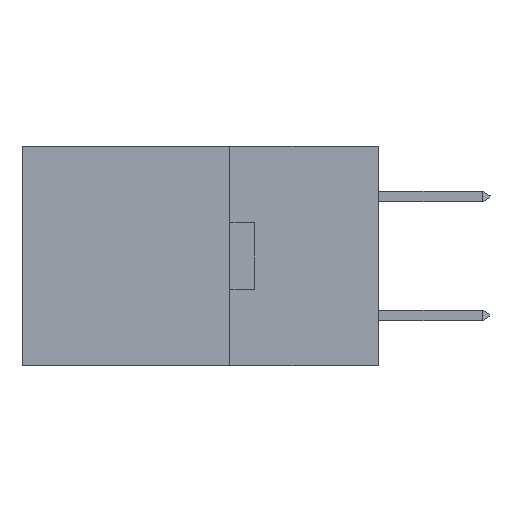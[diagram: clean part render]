
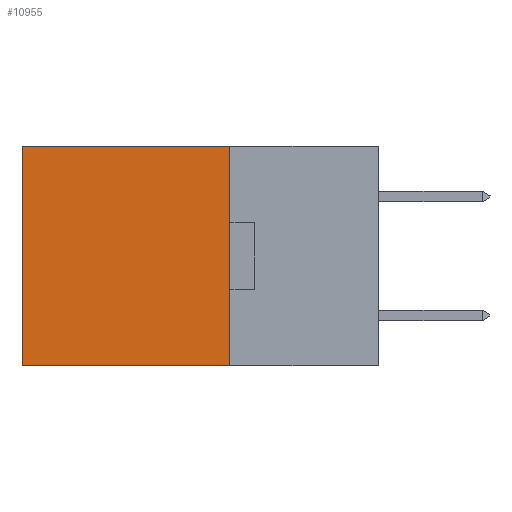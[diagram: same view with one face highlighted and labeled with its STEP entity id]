
A CAD part, left-side view. The second image highlights one B-rep face of the part: STEP entity #10955.
In plain terms, the highlighted planar face has unit normal (-1, 0, 0).
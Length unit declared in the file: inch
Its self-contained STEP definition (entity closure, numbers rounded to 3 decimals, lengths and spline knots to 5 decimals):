
#260 = CARTESIAN_POINT ( 'NONE',  ( 0.2615, 0.6, -0.37 ) ) ;
#2380 = DIRECTION ( 'NONE',  ( 0., 0., -1. ) ) ;
#3137 = CARTESIAN_POINT ( 'NONE',  ( 0.2615, 0.25, -0.37 ) ) ;
#4260 = VECTOR ( 'NONE', #11902, 39.37008 ) ;
#5632 = EDGE_CURVE ( 'NONE', #25134, #18917, #22553, .T. ) ;
#5729 = VECTOR ( 'NONE', #23859, 39.37008 ) ;
#6984 = FACE_OUTER_BOUND ( 'NONE', #23196, .T. ) ;
#8907 = DIRECTION ( 'NONE',  ( 0., 0., -1. ) ) ;
#9344 = ORIENTED_EDGE ( 'NONE', *, *, #13619, .T. ) ;
#9920 = CARTESIAN_POINT ( 'NONE',  ( 0.2615, 0.25, -0.37 ) ) ;
#9975 = ORIENTED_EDGE ( 'NONE', *, *, #25076, .F. ) ;
#10955 = ADVANCED_FACE ( 'NONE', ( #6984 ), #11305, .F. ) ;
#11305 = PLANE ( 'NONE',  #12010 ) ;
#11430 = ORIENTED_EDGE ( 'NONE', *, *, #5632, .T. ) ;
#11448 = CARTESIAN_POINT ( 'NONE',  ( 0.2615, 0.25, -0.37 ) ) ;
#11644 = EDGE_CURVE ( 'NONE', #19443, #21706, #13098, .T. ) ;
#11902 = DIRECTION ( 'NONE',  ( 0., 0., -1. ) ) ;
#12010 = AXIS2_PLACEMENT_3D ( 'NONE', #11448, #20041, #2380 ) ;
#12634 = VECTOR ( 'NONE', #8907, 39.37008 ) ;
#12747 = VECTOR ( 'NONE', #19051, 39.37008 ) ;
#13098 = LINE ( 'NONE', #15105, #5729 ) ;
#13619 = EDGE_CURVE ( 'NONE', #18917, #21706, #19813, .T. ) ;
#14206 = CARTESIAN_POINT ( 'NONE',  ( 0.2615, 0.25, 0. ) ) ;
#15105 = CARTESIAN_POINT ( 'NONE',  ( 0.2615, 0.25, -0.37 ) ) ;
#18917 = VERTEX_POINT ( 'NONE', #23150 ) ;
#19051 = DIRECTION ( 'NONE',  ( 0., 1., 0. ) ) ;
#19443 = VERTEX_POINT ( 'NONE', #9920 ) ;
#19813 = LINE ( 'NONE', #260, #12634 ) ;
#19871 = ORIENTED_EDGE ( 'NONE', *, *, #11644, .F. ) ;
#20041 = DIRECTION ( 'NONE',  ( 1., 0., 0. ) ) ;
#21706 = VERTEX_POINT ( 'NONE', #23542 ) ;
#22553 = LINE ( 'NONE', #25519, #12747 ) ;
#23096 = LINE ( 'NONE', #3137, #4260 ) ;
#23150 = CARTESIAN_POINT ( 'NONE',  ( 0.2615, 0.6, 0. ) ) ;
#23196 = EDGE_LOOP ( 'NONE', ( #9344, #19871, #9975, #11430 ) ) ;
#23542 = CARTESIAN_POINT ( 'NONE',  ( 0.2615, 0.6, -0.37 ) ) ;
#23859 = DIRECTION ( 'NONE',  ( 0., 1., 0. ) ) ;
#25076 = EDGE_CURVE ( 'NONE', #25134, #19443, #23096, .T. ) ;
#25134 = VERTEX_POINT ( 'NONE', #14206 ) ;
#25519 = CARTESIAN_POINT ( 'NONE',  ( 0.2615, 0.25, 0. ) ) ;
